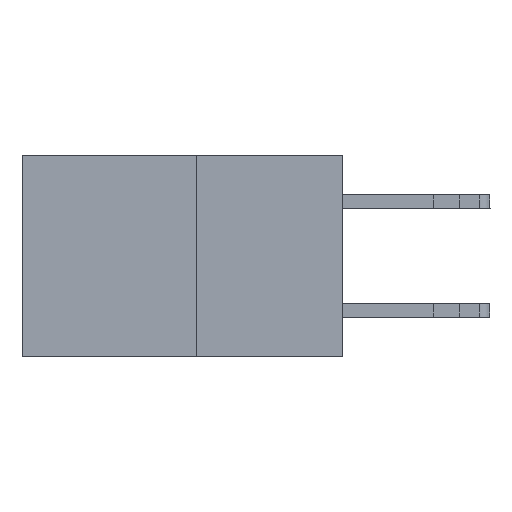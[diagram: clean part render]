
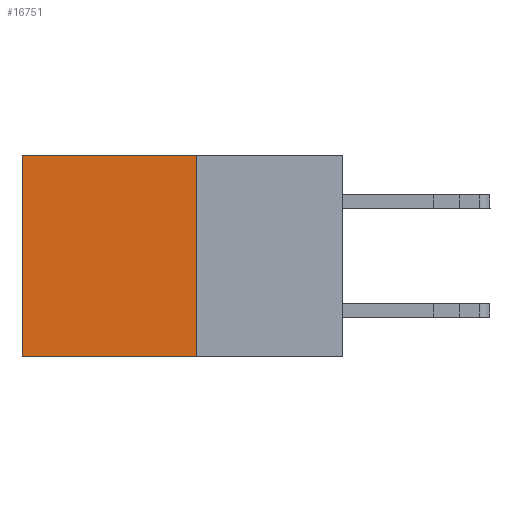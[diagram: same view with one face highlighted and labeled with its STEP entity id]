
A CAD part, left-side view. The second image highlights one B-rep face of the part: STEP entity #16751.
In plain terms, the highlighted planar face has unit normal (-1, 0, 0).
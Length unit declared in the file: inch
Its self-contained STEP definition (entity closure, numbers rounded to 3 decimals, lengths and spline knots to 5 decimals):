
#29 = CARTESIAN_POINT ( 'NONE',  ( 0.277, 0.27, 0. ) ) ;
#1367 = VECTOR ( 'NONE', #2636, 39.37008 ) ;
#1370 = VECTOR ( 'NONE', #9222, 39.37008 ) ;
#1457 = DIRECTION ( 'NONE',  ( 0., 1., 0. ) ) ;
#2382 = CARTESIAN_POINT ( 'NONE',  ( 0.277, 0.27, -0.37 ) ) ;
#2636 = DIRECTION ( 'NONE',  ( 0., 0., -1. ) ) ;
#3121 = LINE ( 'NONE', #11941, #1367 ) ;
#3328 = LINE ( 'NONE', #12827, #16920 ) ;
#3741 = VERTEX_POINT ( 'NONE', #6556 ) ;
#3812 = PLANE ( 'NONE',  #9021 ) ;
#4058 = ORIENTED_EDGE ( 'NONE', *, *, #14896, .T. ) ;
#4229 = FACE_OUTER_BOUND ( 'NONE', #9533, .T. ) ;
#4551 = EDGE_CURVE ( 'NONE', #8325, #5540, #3328, .T. ) ;
#5540 = VERTEX_POINT ( 'NONE', #2382 ) ;
#6556 = CARTESIAN_POINT ( 'NONE',  ( 0.277, 0.59, 0. ) ) ;
#6728 = EDGE_CURVE ( 'NONE', #8325, #3741, #8061, .T. ) ;
#7519 = ORIENTED_EDGE ( 'NONE', *, *, #15656, .F. ) ;
#7846 = DIRECTION ( 'NONE',  ( 1., 0., 0. ) ) ;
#8061 = LINE ( 'NONE', #9845, #1370 ) ;
#8119 = CARTESIAN_POINT ( 'NONE',  ( 0.277, 0.27, -0.37 ) ) ;
#8177 = ORIENTED_EDGE ( 'NONE', *, *, #6728, .T. ) ;
#8325 = VERTEX_POINT ( 'NONE', #29 ) ;
#8335 = LINE ( 'NONE', #8119, #14929 ) ;
#8461 = ORIENTED_EDGE ( 'NONE', *, *, #4551, .F. ) ;
#9021 = AXIS2_PLACEMENT_3D ( 'NONE', #15727, #7846, #16976 ) ;
#9222 = DIRECTION ( 'NONE',  ( 0., 1., 0. ) ) ;
#9533 = EDGE_LOOP ( 'NONE', ( #4058, #7519, #8461, #8177 ) ) ;
#9845 = CARTESIAN_POINT ( 'NONE',  ( 0.277, 0.27, 0. ) ) ;
#11941 = CARTESIAN_POINT ( 'NONE',  ( 0.277, 0.59, -0.37 ) ) ;
#12827 = CARTESIAN_POINT ( 'NONE',  ( 0.277, 0.27, -0.37 ) ) ;
#14368 = DIRECTION ( 'NONE',  ( 0., 0., -1. ) ) ;
#14896 = EDGE_CURVE ( 'NONE', #3741, #16450, #3121, .T. ) ;
#14929 = VECTOR ( 'NONE', #1457, 39.37008 ) ;
#15656 = EDGE_CURVE ( 'NONE', #5540, #16450, #8335, .T. ) ;
#15727 = CARTESIAN_POINT ( 'NONE',  ( 0.277, 0.27, -0.37 ) ) ;
#16188 = CARTESIAN_POINT ( 'NONE',  ( 0.277, 0.59, -0.37 ) ) ;
#16450 = VERTEX_POINT ( 'NONE', #16188 ) ;
#16751 = ADVANCED_FACE ( 'NONE', ( #4229 ), #3812, .F. ) ;
#16920 = VECTOR ( 'NONE', #14368, 39.37008 ) ;
#16976 = DIRECTION ( 'NONE',  ( 0., 0., -1. ) ) ;
